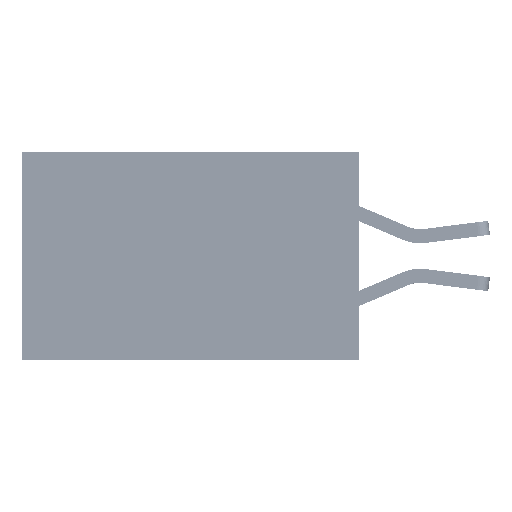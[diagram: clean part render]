
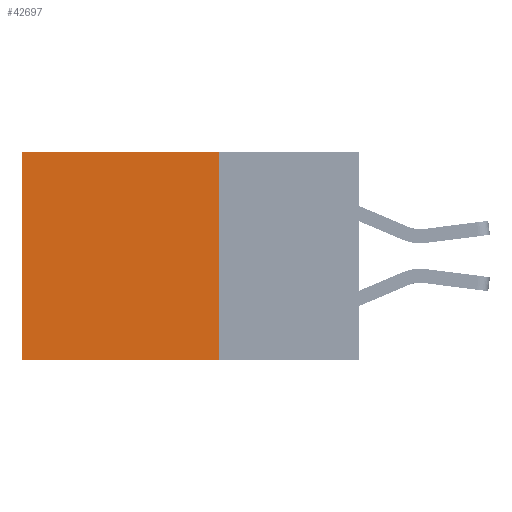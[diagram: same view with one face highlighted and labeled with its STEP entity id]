
A CAD part, left-side view. The second image highlights one B-rep face of the part: STEP entity #42697.
In plain terms, the highlighted planar face has unit normal (-1, 0, 0).
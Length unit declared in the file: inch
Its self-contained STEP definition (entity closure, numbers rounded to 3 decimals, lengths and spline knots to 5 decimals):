
#5196 = LINE ( 'NONE', #38833, #7538 ) ;
#6548 = LINE ( 'NONE', #41375, #7738 ) ;
#7455 = DIRECTION ( 'NONE',  ( 0., 1., 0. ) ) ;
#7538 = VECTOR ( 'NONE', #20121, 39.37008 ) ;
#7738 = VECTOR ( 'NONE', #11569, 39.37008 ) ;
#10203 = CARTESIAN_POINT ( 'NONE',  ( 0.2875, 0.25, 0. ) ) ;
#11569 = DIRECTION ( 'NONE',  ( 0., 1., 0. ) ) ;
#11820 = VERTEX_POINT ( 'NONE', #23222 ) ;
#14656 = VECTOR ( 'NONE', #7455, 39.37008 ) ;
#15068 = ORIENTED_EDGE ( 'NONE', *, *, #16542, .F. ) ;
#15835 = CARTESIAN_POINT ( 'NONE',  ( 0.2875, 0.25, -0.37 ) ) ;
#16261 = EDGE_LOOP ( 'NONE', ( #18774, #15068, #45477, #30532 ) ) ;
#16542 = EDGE_CURVE ( 'NONE', #17706, #11820, #6548, .T. ) ;
#17706 = VERTEX_POINT ( 'NONE', #15835 ) ;
#18345 = EDGE_CURVE ( 'NONE', #34350, #17706, #5196, .T. ) ;
#18774 = ORIENTED_EDGE ( 'NONE', *, *, #41407, .T. ) ;
#19117 = FACE_OUTER_BOUND ( 'NONE', #16261, .T. ) ;
#19335 = DIRECTION ( 'NONE',  ( 0., 0., -1. ) ) ;
#20121 = DIRECTION ( 'NONE',  ( 0., 0., -1. ) ) ;
#23222 = CARTESIAN_POINT ( 'NONE',  ( 0.2875, 0.6, -0.37 ) ) ;
#26192 = AXIS2_PLACEMENT_3D ( 'NONE', #48205, #30679, #29495 ) ;
#27798 = EDGE_CURVE ( 'NONE', #34350, #33976, #47290, .T. ) ;
#29495 = DIRECTION ( 'NONE',  ( 0., 0., -1. ) ) ;
#30527 = PLANE ( 'NONE',  #26192 ) ;
#30532 = ORIENTED_EDGE ( 'NONE', *, *, #27798, .T. ) ;
#30679 = DIRECTION ( 'NONE',  ( 1., 0., 0. ) ) ;
#33877 = CARTESIAN_POINT ( 'NONE',  ( 0.2875, 0.25, 0. ) ) ;
#33976 = VERTEX_POINT ( 'NONE', #41655 ) ;
#34350 = VERTEX_POINT ( 'NONE', #10203 ) ;
#34421 = VECTOR ( 'NONE', #19335, 39.37008 ) ;
#38833 = CARTESIAN_POINT ( 'NONE',  ( 0.2875, 0.25, 0. ) ) ;
#41375 = CARTESIAN_POINT ( 'NONE',  ( 0.2875, 0.25, -0.37 ) ) ;
#41407 = EDGE_CURVE ( 'NONE', #33976, #11820, #46056, .T. ) ;
#41655 = CARTESIAN_POINT ( 'NONE',  ( 0.2875, 0.6, 0. ) ) ;
#42697 = ADVANCED_FACE ( 'NONE', ( #19117 ), #30527, .F. ) ;
#44749 = CARTESIAN_POINT ( 'NONE',  ( 0.2875, 0.6, 0. ) ) ;
#45477 = ORIENTED_EDGE ( 'NONE', *, *, #18345, .F. ) ;
#46056 = LINE ( 'NONE', #44749, #34421 ) ;
#47290 = LINE ( 'NONE', #33877, #14656 ) ;
#48205 = CARTESIAN_POINT ( 'NONE',  ( 0.2875, 0.25, 0. ) ) ;
